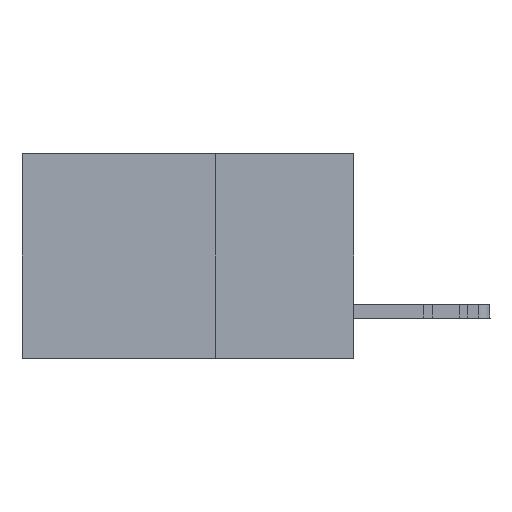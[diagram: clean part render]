
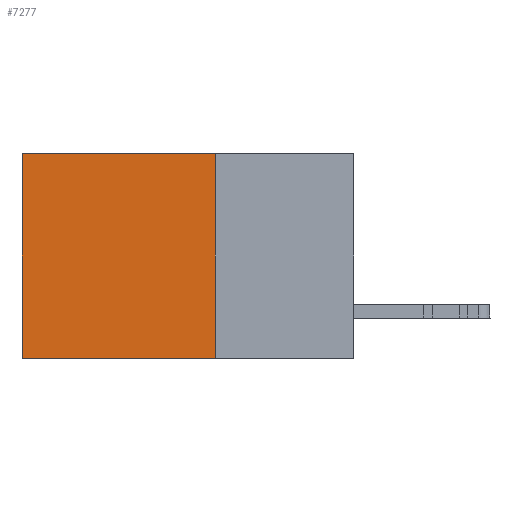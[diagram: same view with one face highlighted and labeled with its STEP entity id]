
A CAD part, left-side view. The second image highlights one B-rep face of the part: STEP entity #7277.
In plain terms, the highlighted planar face has unit normal (-1, 0, 0).
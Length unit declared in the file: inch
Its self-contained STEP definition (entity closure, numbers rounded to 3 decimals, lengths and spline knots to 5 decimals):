
#461 = EDGE_CURVE ( 'NONE', #18885, #36936, #13296, .T. ) ;
#1384 = EDGE_LOOP ( 'NONE', ( #42235, #13846, #1720, #36264 ) ) ;
#1720 = ORIENTED_EDGE ( 'NONE', *, *, #461, .F. ) ;
#4206 = DIRECTION ( 'NONE',  ( 0., 1., 0. ) ) ;
#4586 = CARTESIAN_POINT ( 'NONE',  ( 0.2875, 0.25, 0. ) ) ;
#5740 = VECTOR ( 'NONE', #4206, 39.37008 ) ;
#6397 = PLANE ( 'NONE',  #28320 ) ;
#7277 = ADVANCED_FACE ( 'NONE', ( #20197 ), #6397, .F. ) ;
#8007 = CARTESIAN_POINT ( 'NONE',  ( 0.2875, 0.6, 0. ) ) ;
#8171 = CARTESIAN_POINT ( 'NONE',  ( 0.2875, 0.6, -0.37 ) ) ;
#8952 = CARTESIAN_POINT ( 'NONE',  ( 0.2875, 0.25, -0.37 ) ) ;
#9833 = CARTESIAN_POINT ( 'NONE',  ( 0.2875, 0.25, 0. ) ) ;
#9947 = LINE ( 'NONE', #4586, #43265 ) ;
#10449 = VECTOR ( 'NONE', #39569, 39.37008 ) ;
#13296 = LINE ( 'NONE', #9833, #16515 ) ;
#13308 = DIRECTION ( 'NONE',  ( 0., 0., -1. ) ) ;
#13846 = ORIENTED_EDGE ( 'NONE', *, *, #18452, .F. ) ;
#16515 = VECTOR ( 'NONE', #41485, 39.37008 ) ;
#17576 = CARTESIAN_POINT ( 'NONE',  ( 0.2875, 0.25, -0.37 ) ) ;
#18452 = EDGE_CURVE ( 'NONE', #36936, #20923, #32033, .T. ) ;
#18885 = VERTEX_POINT ( 'NONE', #37919 ) ;
#20197 = FACE_OUTER_BOUND ( 'NONE', #1384, .T. ) ;
#20923 = VERTEX_POINT ( 'NONE', #8171 ) ;
#22892 = LINE ( 'NONE', #28923, #10449 ) ;
#27387 = EDGE_CURVE ( 'NONE', #18885, #27843, #9947, .T. ) ;
#27843 = VERTEX_POINT ( 'NONE', #8007 ) ;
#28320 = AXIS2_PLACEMENT_3D ( 'NONE', #41349, #37765, #13308 ) ;
#28633 = DIRECTION ( 'NONE',  ( 0., 1., 0. ) ) ;
#28923 = CARTESIAN_POINT ( 'NONE',  ( 0.2875, 0.6, 0. ) ) ;
#32033 = LINE ( 'NONE', #17576, #5740 ) ;
#36264 = ORIENTED_EDGE ( 'NONE', *, *, #27387, .T. ) ;
#36936 = VERTEX_POINT ( 'NONE', #8952 ) ;
#37765 = DIRECTION ( 'NONE',  ( 1., 0., 0. ) ) ;
#37919 = CARTESIAN_POINT ( 'NONE',  ( 0.2875, 0.25, 0. ) ) ;
#39569 = DIRECTION ( 'NONE',  ( 0., 0., -1. ) ) ;
#41349 = CARTESIAN_POINT ( 'NONE',  ( 0.2875, 0.25, 0. ) ) ;
#41485 = DIRECTION ( 'NONE',  ( 0., 0., -1. ) ) ;
#42235 = ORIENTED_EDGE ( 'NONE', *, *, #44316, .T. ) ;
#43265 = VECTOR ( 'NONE', #28633, 39.37008 ) ;
#44316 = EDGE_CURVE ( 'NONE', #27843, #20923, #22892, .T. ) ;
